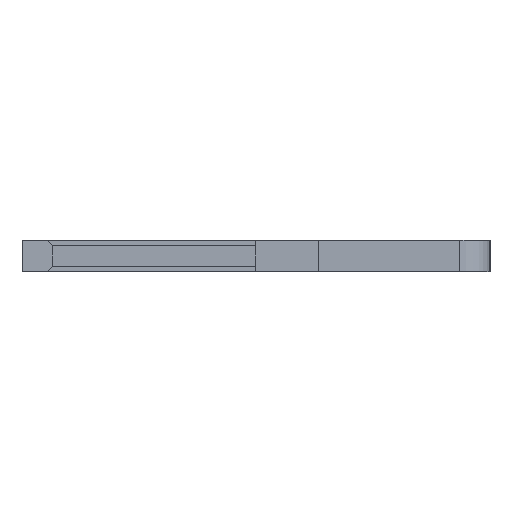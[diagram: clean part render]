
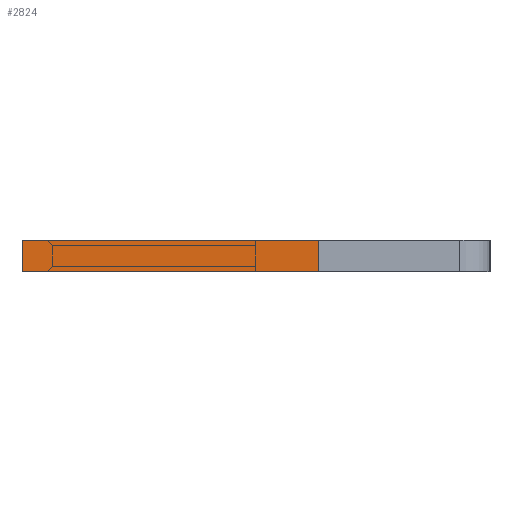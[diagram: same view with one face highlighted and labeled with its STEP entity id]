
A CAD part, left-side view. The second image highlights one B-rep face of the part: STEP entity #2824.
In plain terms, the highlighted face is planar.
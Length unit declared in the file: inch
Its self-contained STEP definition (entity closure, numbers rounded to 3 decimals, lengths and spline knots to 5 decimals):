
#65 = EDGE_CURVE ( 'NONE', #1817, #3617, #4062, .T. ) ;
#80 = CARTESIAN_POINT ( 'NONE',  ( -0.01, 0.15, -0.04 ) ) ;
#243 = VECTOR ( 'NONE', #495, 39.37008 ) ;
#372 = CARTESIAN_POINT ( 'NONE',  ( 0.01, 0.15, -0.04 ) ) ;
#485 = FACE_OUTER_BOUND ( 'NONE', #1714, .T. ) ;
#495 = DIRECTION ( 'NONE',  ( -1., 0., 0. ) ) ;
#631 = ORIENTED_EDGE ( 'NONE', *, *, #3952, .T. ) ;
#776 = VERTEX_POINT ( 'NONE', #3022 ) ;
#825 = EDGE_CURVE ( 'NONE', #1169, #776, #2665, .T. ) ;
#1169 = VERTEX_POINT ( 'NONE', #3403 ) ;
#1243 = VECTOR ( 'NONE', #2898, 39.37008 ) ;
#1267 = ORIENTED_EDGE ( 'NONE', *, *, #65, .F. ) ;
#1409 = PLANE ( 'NONE',  #3565 ) ;
#1410 = CARTESIAN_POINT ( 'NONE',  ( 0.01, 0.15, -0.04 ) ) ;
#1714 = EDGE_LOOP ( 'NONE', ( #631, #1267, #3353, #3958 ) ) ;
#1782 = DIRECTION ( 'NONE',  ( 0., 0., 1. ) ) ;
#1817 = VERTEX_POINT ( 'NONE', #1410 ) ;
#1964 = VECTOR ( 'NONE', #3039, 39.37008 ) ;
#2345 = LINE ( 'NONE', #2810, #4266 ) ;
#2352 = DIRECTION ( 'NONE',  ( 0., 1., 0. ) ) ;
#2452 = DIRECTION ( 'NONE',  ( 1., 0., 0. ) ) ;
#2628 = CARTESIAN_POINT ( 'NONE',  ( 0.01, -0.04, -0.04 ) ) ;
#2665 = LINE ( 'NONE', #2628, #1964 ) ;
#2810 = CARTESIAN_POINT ( 'NONE',  ( -0.01, 0.15, -0.04 ) ) ;
#2824 = ADVANCED_FACE ( 'NONE', ( #485 ), #1409, .F. ) ;
#2898 = DIRECTION ( 'NONE',  ( 0., 1., 0. ) ) ;
#2903 = CARTESIAN_POINT ( 'NONE',  ( 0.01, 0.15, -0.04 ) ) ;
#3022 = CARTESIAN_POINT ( 'NONE',  ( -0.01, -0.04, -0.04 ) ) ;
#3039 = DIRECTION ( 'NONE',  ( -1., 0., 0. ) ) ;
#3228 = CARTESIAN_POINT ( 'NONE',  ( 0.01, 0.15, -0.04 ) ) ;
#3240 = EDGE_CURVE ( 'NONE', #1169, #1817, #3426, .T. ) ;
#3353 = ORIENTED_EDGE ( 'NONE', *, *, #3240, .F. ) ;
#3403 = CARTESIAN_POINT ( 'NONE',  ( 0.01, -0.04, -0.04 ) ) ;
#3426 = LINE ( 'NONE', #3228, #1243 ) ;
#3565 = AXIS2_PLACEMENT_3D ( 'NONE', #372, #1782, #2452 ) ;
#3617 = VERTEX_POINT ( 'NONE', #80 ) ;
#3952 = EDGE_CURVE ( 'NONE', #776, #3617, #2345, .T. ) ;
#3958 = ORIENTED_EDGE ( 'NONE', *, *, #825, .T. ) ;
#4062 = LINE ( 'NONE', #2903, #243 ) ;
#4266 = VECTOR ( 'NONE', #2352, 39.37008 ) ;
